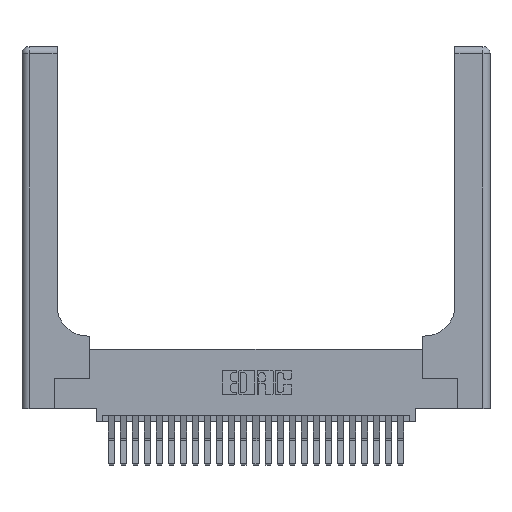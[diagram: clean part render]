
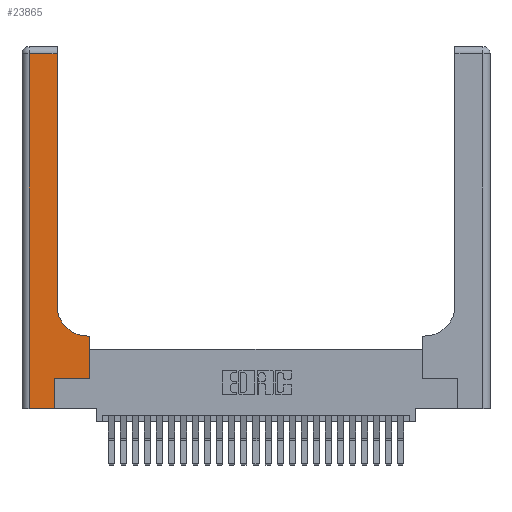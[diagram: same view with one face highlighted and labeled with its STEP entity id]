
A CAD part, top view. The second image highlights one B-rep face of the part: STEP entity #23865.
In plain terms, the highlighted planar face has unit normal (0, 0, 1).
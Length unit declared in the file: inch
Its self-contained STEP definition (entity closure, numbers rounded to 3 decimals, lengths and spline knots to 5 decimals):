
#493 = ORIENTED_EDGE ( 'NONE', *, *, #22986, .T. ) ;
#761 = ORIENTED_EDGE ( 'NONE', *, *, #8311, .T. ) ;
#1196 = CARTESIAN_POINT ( 'NONE',  ( 0.2915, 0.85, 0.37 ) ) ;
#2090 = CARTESIAN_POINT ( 'NONE',  ( 0.2915, 3., 0.37 ) ) ;
#2517 = EDGE_CURVE ( 'NONE', #6776, #19621, #9861, .T. ) ;
#2521 = EDGE_CURVE ( 'NONE', #6210, #13227, #26328, .T. ) ;
#2679 = VERTEX_POINT ( 'NONE', #22811 ) ;
#2833 = LINE ( 'NONE', #25041, #9441 ) ;
#3848 = ORIENTED_EDGE ( 'NONE', *, *, #2517, .T. ) ;
#3904 = ORIENTED_EDGE ( 'NONE', *, *, #22789, .T. ) ;
#4679 = CARTESIAN_POINT ( 'NONE',  ( 0.5585, 0.25, 0.37 ) ) ;
#5029 = DIRECTION ( 'NONE',  ( -1., 0., 0. ) ) ;
#5106 = VERTEX_POINT ( 'NONE', #4679 ) ;
#5283 = DIRECTION ( 'NONE',  ( 1., 0., 0. ) ) ;
#6103 = LINE ( 'NONE', #15644, #26206 ) ;
#6210 = VERTEX_POINT ( 'NONE', #24147 ) ;
#6277 = CARTESIAN_POINT ( 'NONE',  ( 0.269, 0., 0.37 ) ) ;
#6633 = DIRECTION ( 'NONE',  ( 0., 1., 0. ) ) ;
#6776 = VERTEX_POINT ( 'NONE', #1196 ) ;
#7543 = CARTESIAN_POINT ( 'NONE',  ( 0., 2.94, 0.37 ) ) ;
#8311 = EDGE_CURVE ( 'NONE', #19621, #11125, #25567, .T. ) ;
#8343 = EDGE_CURVE ( 'NONE', #12702, #13491, #6103, .T. ) ;
#8723 = LINE ( 'NONE', #19295, #22282 ) ;
#9441 = VECTOR ( 'NONE', #14713, 39.37008 ) ;
#9861 = LINE ( 'NONE', #2090, #27325 ) ;
#10376 = EDGE_CURVE ( 'NONE', #11125, #2679, #23805, .T. ) ;
#10835 = AXIS2_PLACEMENT_3D ( 'NONE', #26030, #26120, #21732 ) ;
#11125 = VERTEX_POINT ( 'NONE', #19442 ) ;
#12499 = ORIENTED_EDGE ( 'NONE', *, *, #10376, .T. ) ;
#12702 = VERTEX_POINT ( 'NONE', #13503 ) ;
#13227 = VERTEX_POINT ( 'NONE', #20483 ) ;
#13253 = CARTESIAN_POINT ( 'NONE',  ( 0.2915, 2.94, 0.37 ) ) ;
#13491 = VERTEX_POINT ( 'NONE', #25251 ) ;
#13503 = CARTESIAN_POINT ( 'NONE',  ( 0.5585, 0.6, 0.37 ) ) ;
#14400 = VECTOR ( 'NONE', #5283, 39.37008 ) ;
#14713 = DIRECTION ( 'NONE',  ( 0., 1., 0. ) ) ;
#15644 = CARTESIAN_POINT ( 'NONE',  ( 0.2915, 0.6, 0.37 ) ) ;
#15645 = EDGE_LOOP ( 'NONE', ( #3848, #761, #12499, #493, #26963, #21392, #22301, #16420, #3904 ) ) ;
#15666 = CIRCLE ( 'NONE', #10835, 0.25 ) ;
#16420 = ORIENTED_EDGE ( 'NONE', *, *, #8343, .T. ) ;
#16853 = DIRECTION ( 'NONE',  ( 0., 1., 0. ) ) ;
#16862 = EDGE_CURVE ( 'NONE', #13227, #5106, #23644, .T. ) ;
#17549 = EDGE_CURVE ( 'NONE', #5106, #12702, #2833, .T. ) ;
#17639 = PLANE ( 'NONE',  #26761 ) ;
#17965 = FACE_OUTER_BOUND ( 'NONE', #15645, .T. ) ;
#18126 = DIRECTION ( 'NONE',  ( -1., 0., 0. ) ) ;
#18202 = VECTOR ( 'NONE', #27128, 39.37008 ) ;
#19295 = CARTESIAN_POINT ( 'NONE',  ( 0., 0., 0.37 ) ) ;
#19442 = CARTESIAN_POINT ( 'NONE',  ( 0.06, 2.94, 0.37 ) ) ;
#19564 = DIRECTION ( 'NONE',  ( 0., 0., -1. ) ) ;
#19621 = VERTEX_POINT ( 'NONE', #13253 ) ;
#20011 = CARTESIAN_POINT ( 'NONE',  ( 0.269, 0.25, 0.37 ) ) ;
#20061 = VECTOR ( 'NONE', #6633, 39.37008 ) ;
#20483 = CARTESIAN_POINT ( 'NONE',  ( 0.269, 0.25, 0.37 ) ) ;
#21392 = ORIENTED_EDGE ( 'NONE', *, *, #16862, .T. ) ;
#21732 = DIRECTION ( 'NONE',  ( 1., 0., 0. ) ) ;
#22113 = DIRECTION ( 'NONE',  ( -1., 0., 0. ) ) ;
#22282 = VECTOR ( 'NONE', #23208, 39.37008 ) ;
#22301 = ORIENTED_EDGE ( 'NONE', *, *, #17549, .T. ) ;
#22789 = EDGE_CURVE ( 'NONE', #13491, #6776, #15666, .T. ) ;
#22811 = CARTESIAN_POINT ( 'NONE',  ( 0.06, 0., 0.37 ) ) ;
#22986 = EDGE_CURVE ( 'NONE', #2679, #6210, #8723, .T. ) ;
#23017 = CARTESIAN_POINT ( 'NONE',  ( 0.06, 3., 0.37 ) ) ;
#23208 = DIRECTION ( 'NONE',  ( 1., 0., 0. ) ) ;
#23644 = LINE ( 'NONE', #20011, #14400 ) ;
#23805 = LINE ( 'NONE', #23017, #18202 ) ;
#23865 = ADVANCED_FACE ( 'NONE', ( #17965 ), #17639, .F. ) ;
#24147 = CARTESIAN_POINT ( 'NONE',  ( 0.269, 0., 0.37 ) ) ;
#24573 = VECTOR ( 'NONE', #22113, 39.37008 ) ;
#25041 = CARTESIAN_POINT ( 'NONE',  ( 0.5585, 0.25, 0.37 ) ) ;
#25251 = CARTESIAN_POINT ( 'NONE',  ( 0.5415, 0.6, 0.37 ) ) ;
#25567 = LINE ( 'NONE', #7543, #24573 ) ;
#26030 = CARTESIAN_POINT ( 'NONE',  ( 0.5415, 0.85, 0.37 ) ) ;
#26120 = DIRECTION ( 'NONE',  ( 0., 0., -1. ) ) ;
#26203 = CARTESIAN_POINT ( 'NONE',  ( 0., 3., 0.37 ) ) ;
#26206 = VECTOR ( 'NONE', #18126, 39.37008 ) ;
#26328 = LINE ( 'NONE', #6277, #20061 ) ;
#26761 = AXIS2_PLACEMENT_3D ( 'NONE', #26203, #19564, #5029 ) ;
#26963 = ORIENTED_EDGE ( 'NONE', *, *, #2521, .T. ) ;
#27128 = DIRECTION ( 'NONE',  ( 0., -1., 0. ) ) ;
#27325 = VECTOR ( 'NONE', #16853, 39.37008 ) ;
